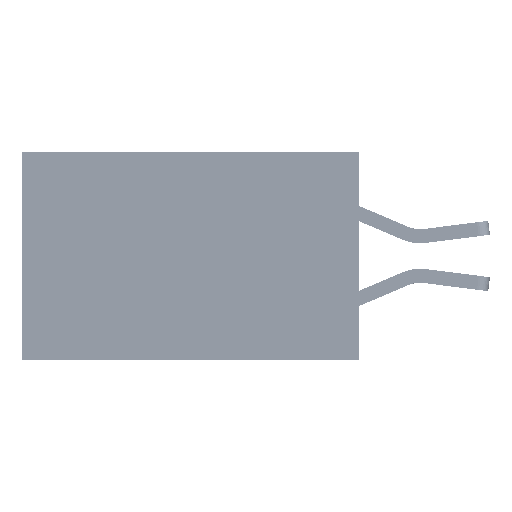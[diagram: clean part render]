
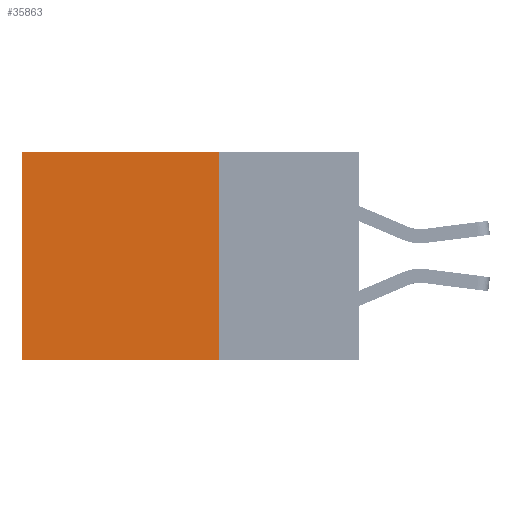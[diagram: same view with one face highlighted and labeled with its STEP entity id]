
A CAD part, left-side view. The second image highlights one B-rep face of the part: STEP entity #35863.
In plain terms, the highlighted planar face has unit normal (-1, 0, 0).
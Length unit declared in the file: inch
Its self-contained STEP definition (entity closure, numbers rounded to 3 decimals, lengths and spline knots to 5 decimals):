
#2021 = VERTEX_POINT ( 'NONE', #39328 ) ;
#3761 = DIRECTION ( 'NONE',  ( 0., 1., 0. ) ) ;
#5037 = VECTOR ( 'NONE', #13331, 39.37008 ) ;
#5296 = VECTOR ( 'NONE', #3761, 39.37008 ) ;
#5572 = DIRECTION ( 'NONE',  ( 0., 1., 0. ) ) ;
#7178 = EDGE_CURVE ( 'NONE', #9363, #11773, #24887, .T. ) ;
#8325 = LINE ( 'NONE', #38389, #14200 ) ;
#9363 = VERTEX_POINT ( 'NONE', #34803 ) ;
#11522 = FACE_OUTER_BOUND ( 'NONE', #31998, .T. ) ;
#11773 = VERTEX_POINT ( 'NONE', #20692 ) ;
#13331 = DIRECTION ( 'NONE',  ( 0., 0., -1. ) ) ;
#14200 = VECTOR ( 'NONE', #42123, 39.37008 ) ;
#14898 = CARTESIAN_POINT ( 'NONE',  ( 0.2875, 0.25, 0. ) ) ;
#19609 = ORIENTED_EDGE ( 'NONE', *, *, #7178, .T. ) ;
#19820 = DIRECTION ( 'NONE',  ( 0., 0., -1. ) ) ;
#20692 = CARTESIAN_POINT ( 'NONE',  ( 0.2875, 0.6, -0.37 ) ) ;
#21089 = LINE ( 'NONE', #39230, #37916 ) ;
#23880 = EDGE_CURVE ( 'NONE', #2021, #11773, #21089, .T. ) ;
#24887 = LINE ( 'NONE', #35549, #5037 ) ;
#26010 = ORIENTED_EDGE ( 'NONE', *, *, #28355, .F. ) ;
#26516 = CARTESIAN_POINT ( 'NONE',  ( 0.2875, 0.25, 0. ) ) ;
#27531 = CARTESIAN_POINT ( 'NONE',  ( 0.2875, 0.25, 0. ) ) ;
#28355 = EDGE_CURVE ( 'NONE', #42445, #2021, #8325, .T. ) ;
#31998 = EDGE_LOOP ( 'NONE', ( #19609, #38262, #26010, #41864 ) ) ;
#32012 = LINE ( 'NONE', #14898, #5296 ) ;
#34803 = CARTESIAN_POINT ( 'NONE',  ( 0.2875, 0.6, 0. ) ) ;
#35549 = CARTESIAN_POINT ( 'NONE',  ( 0.2875, 0.6, 0. ) ) ;
#35863 = ADVANCED_FACE ( 'NONE', ( #11522 ), #46017, .F. ) ;
#37916 = VECTOR ( 'NONE', #5572, 39.37008 ) ;
#38262 = ORIENTED_EDGE ( 'NONE', *, *, #23880, .F. ) ;
#38285 = DIRECTION ( 'NONE',  ( 1., 0., 0. ) ) ;
#38389 = CARTESIAN_POINT ( 'NONE',  ( 0.2875, 0.25, 0. ) ) ;
#39230 = CARTESIAN_POINT ( 'NONE',  ( 0.2875, 0.25, -0.37 ) ) ;
#39328 = CARTESIAN_POINT ( 'NONE',  ( 0.2875, 0.25, -0.37 ) ) ;
#40501 = AXIS2_PLACEMENT_3D ( 'NONE', #27531, #38285, #19820 ) ;
#41864 = ORIENTED_EDGE ( 'NONE', *, *, #46832, .T. ) ;
#42123 = DIRECTION ( 'NONE',  ( 0., 0., -1. ) ) ;
#42445 = VERTEX_POINT ( 'NONE', #26516 ) ;
#46017 = PLANE ( 'NONE',  #40501 ) ;
#46832 = EDGE_CURVE ( 'NONE', #42445, #9363, #32012, .T. ) ;
